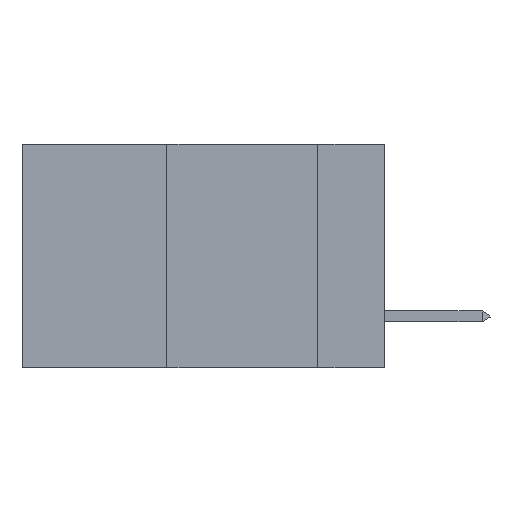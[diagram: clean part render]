
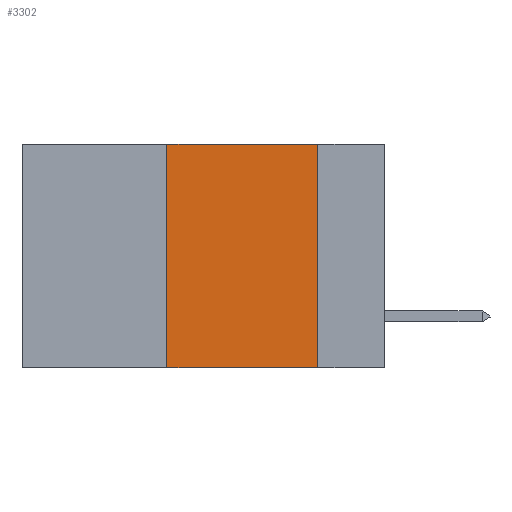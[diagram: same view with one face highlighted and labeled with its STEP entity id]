
A CAD part, left-side view. The second image highlights one B-rep face of the part: STEP entity #3302.
In plain terms, the highlighted planar face has unit normal (-1, 0, 0).
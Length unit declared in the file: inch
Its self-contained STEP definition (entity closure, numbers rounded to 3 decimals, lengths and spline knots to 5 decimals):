
#452 = AXIS2_PLACEMENT_3D ( 'NONE', #7755, #7920, #6843 ) ;
#731 = VECTOR ( 'NONE', #5693, 39.37008 ) ;
#882 = PLANE ( 'NONE',  #452 ) ;
#914 = ORIENTED_EDGE ( 'NONE', *, *, #4485, .F. ) ;
#2114 = DIRECTION ( 'NONE',  ( 0., 0., 1. ) ) ;
#2277 = VERTEX_POINT ( 'NONE', #6547 ) ;
#3067 = CARTESIAN_POINT ( 'NONE',  ( 0., 0.11, -0.37 ) ) ;
#3084 = ORIENTED_EDGE ( 'NONE', *, *, #3348, .F. ) ;
#3182 = CARTESIAN_POINT ( 'NONE',  ( 0., 0.36, 0. ) ) ;
#3256 = FACE_OUTER_BOUND ( 'NONE', #7274, .T. ) ;
#3302 = ADVANCED_FACE ( 'NONE', ( #3256 ), #882, .F. ) ;
#3348 = EDGE_CURVE ( 'NONE', #7824, #12240, #4354, .T. ) ;
#3370 = CARTESIAN_POINT ( 'NONE',  ( 0., 0.11, 0. ) ) ;
#4354 = LINE ( 'NONE', #3370, #6524 ) ;
#4485 = EDGE_CURVE ( 'NONE', #11527, #2277, #10769, .T. ) ;
#4746 = CARTESIAN_POINT ( 'NONE',  ( 0., 0.6, -0.37 ) ) ;
#5038 = ORIENTED_EDGE ( 'NONE', *, *, #8230, .F. ) ;
#5605 = LINE ( 'NONE', #5919, #10210 ) ;
#5693 = DIRECTION ( 'NONE',  ( 0., -1., 0. ) ) ;
#5919 = CARTESIAN_POINT ( 'NONE',  ( 0., 0.6, 0. ) ) ;
#6384 = LINE ( 'NONE', #4746, #731 ) ;
#6524 = VECTOR ( 'NONE', #8355, 39.37008 ) ;
#6547 = CARTESIAN_POINT ( 'NONE',  ( 0., 0.36, 0. ) ) ;
#6843 = DIRECTION ( 'NONE',  ( 0., 0., -1. ) ) ;
#7274 = EDGE_LOOP ( 'NONE', ( #3084, #5038, #914, #11513 ) ) ;
#7679 = EDGE_CURVE ( 'NONE', #11527, #12240, #6384, .T. ) ;
#7755 = CARTESIAN_POINT ( 'NONE',  ( 0., 0.6, 0. ) ) ;
#7824 = VERTEX_POINT ( 'NONE', #11734 ) ;
#7853 = DIRECTION ( 'NONE',  ( 0., -1., 0. ) ) ;
#7920 = DIRECTION ( 'NONE',  ( 1., 0., 0. ) ) ;
#8230 = EDGE_CURVE ( 'NONE', #2277, #7824, #5605, .T. ) ;
#8355 = DIRECTION ( 'NONE',  ( 0., 0., -1. ) ) ;
#9041 = CARTESIAN_POINT ( 'NONE',  ( 0., 0.36, -0.37 ) ) ;
#10210 = VECTOR ( 'NONE', #7853, 39.37008 ) ;
#10306 = VECTOR ( 'NONE', #2114, 39.37008 ) ;
#10769 = LINE ( 'NONE', #3182, #10306 ) ;
#11513 = ORIENTED_EDGE ( 'NONE', *, *, #7679, .T. ) ;
#11527 = VERTEX_POINT ( 'NONE', #9041 ) ;
#11734 = CARTESIAN_POINT ( 'NONE',  ( 0., 0.11, 0. ) ) ;
#12240 = VERTEX_POINT ( 'NONE', #3067 ) ;
